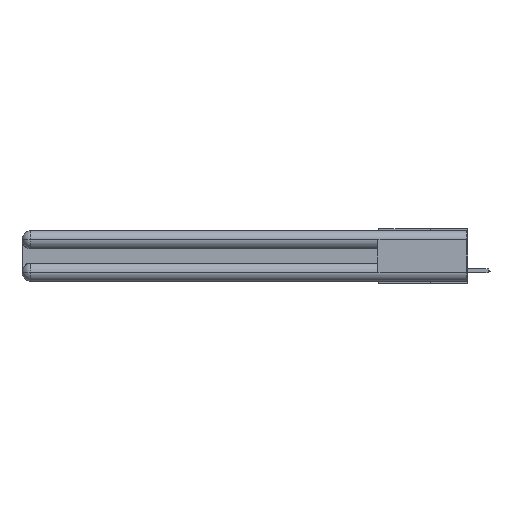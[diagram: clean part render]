
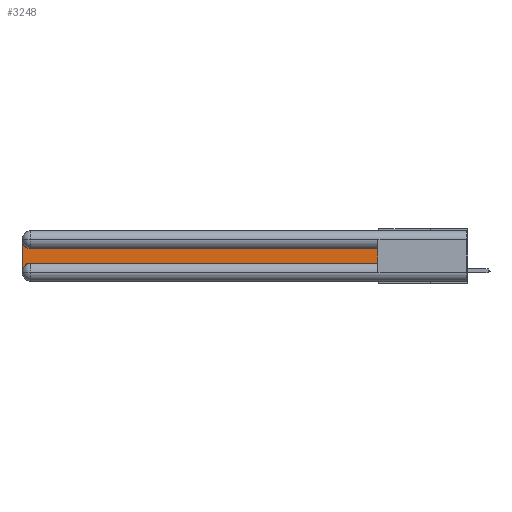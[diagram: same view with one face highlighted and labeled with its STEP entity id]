
A CAD part, left-side view. The second image highlights one B-rep face of the part: STEP entity #3248.
In plain terms, the highlighted planar face has unit normal (-1, 0, 0).
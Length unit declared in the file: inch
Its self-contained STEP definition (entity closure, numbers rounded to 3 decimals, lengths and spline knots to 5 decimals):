
#454 = CARTESIAN_POINT ( 'NONE',  ( 0.075, 3., -0.2775 ) ) ;
#665 = DIRECTION ( 'NONE',  ( 0., -1., 0. ) ) ;
#1036 = DIRECTION ( 'NONE',  ( 0., 1., 0. ) ) ;
#2066 = CARTESIAN_POINT ( 'NONE',  ( 0.075, 2.94, -0.1225 ) ) ;
#2293 = DIRECTION ( 'NONE',  ( 1., 0., 0. ) ) ;
#2367 = EDGE_CURVE ( 'NONE', #18410, #32623, #33781, .T. ) ;
#3248 = ADVANCED_FACE ( 'NONE', ( #12074 ), #4738, .F. ) ;
#3648 = CARTESIAN_POINT ( 'NONE',  ( 0.075, 2.94, -0.0625 ) ) ;
#4433 = DIRECTION ( 'NONE',  ( 0., 0., -1. ) ) ;
#4738 = PLANE ( 'NONE',  #27970 ) ;
#5517 = CARTESIAN_POINT ( 'NONE',  ( 0.075, 2.94, -0.2775 ) ) ;
#6351 = EDGE_CURVE ( 'NONE', #13117, #14638, #25207, .T. ) ;
#6501 = LINE ( 'NONE', #11069, #33966 ) ;
#7961 = CARTESIAN_POINT ( 'NONE',  ( 0.075, 0.6, -0.1225 ) ) ;
#9900 = CARTESIAN_POINT ( 'NONE',  ( 0.075, 3., -0.0625 ) ) ;
#10849 = LINE ( 'NONE', #24907, #33759 ) ;
#11069 = CARTESIAN_POINT ( 'NONE',  ( 0.075, 0.6, -0.2175 ) ) ;
#12074 = FACE_OUTER_BOUND ( 'NONE', #20539, .T. ) ;
#12689 = EDGE_CURVE ( 'NONE', #16022, #32002, #6501, .T. ) ;
#13117 = VERTEX_POINT ( 'NONE', #2066 ) ;
#13530 = ORIENTED_EDGE ( 'NONE', *, *, #12689, .T. ) ;
#14153 = VECTOR ( 'NONE', #27728, 39.37008 ) ;
#14638 = VERTEX_POINT ( 'NONE', #9900 ) ;
#15574 = CARTESIAN_POINT ( 'NONE',  ( 0.075, 3., -0.1225 ) ) ;
#16022 = VERTEX_POINT ( 'NONE', #25966 ) ;
#16686 = DIRECTION ( 'NONE',  ( 0., 0., 1. ) ) ;
#18410 = VERTEX_POINT ( 'NONE', #454 ) ;
#20134 = ORIENTED_EDGE ( 'NONE', *, *, #30797, .T. ) ;
#20539 = EDGE_LOOP ( 'NONE', ( #21805, #30813, #20134, #25543, #29751, #13530 ) ) ;
#21438 = DIRECTION ( 'NONE',  ( 0., 0., -1. ) ) ;
#21559 = DIRECTION ( 'NONE',  ( 1., 0., 0. ) ) ;
#21805 = ORIENTED_EDGE ( 'NONE', *, *, #28909, .T. ) ;
#23029 = VECTOR ( 'NONE', #665, 39.37008 ) ;
#23336 = DIRECTION ( 'NONE',  ( 0., 0., -1. ) ) ;
#24907 = CARTESIAN_POINT ( 'NONE',  ( 0.075, 0.6, -0.1225 ) ) ;
#25207 = CIRCLE ( 'NONE', #30865, 0.06 ) ;
#25400 = CARTESIAN_POINT ( 'NONE',  ( 0.075, 3., -0.2175 ) ) ;
#25543 = ORIENTED_EDGE ( 'NONE', *, *, #2367, .T. ) ;
#25966 = CARTESIAN_POINT ( 'NONE',  ( 0.075, 0.6, -0.2175 ) ) ;
#26603 = CARTESIAN_POINT ( 'NONE',  ( 0.075, 0.6, -0.2175 ) ) ;
#26721 = CARTESIAN_POINT ( 'NONE',  ( 0.075, 2.94, -0.2175 ) ) ;
#27628 = LINE ( 'NONE', #26603, #23029 ) ;
#27728 = DIRECTION ( 'NONE',  ( 0., 0., -1. ) ) ;
#27970 = AXIS2_PLACEMENT_3D ( 'NONE', #15574, #2293, #23336 ) ;
#28297 = DIRECTION ( 'NONE',  ( 1., 0., 0. ) ) ;
#28831 = AXIS2_PLACEMENT_3D ( 'NONE', #5517, #21559, #21438 ) ;
#28909 = EDGE_CURVE ( 'NONE', #32002, #13117, #10849, .T. ) ;
#29490 = LINE ( 'NONE', #25400, #14153 ) ;
#29751 = ORIENTED_EDGE ( 'NONE', *, *, #33095, .T. ) ;
#30797 = EDGE_CURVE ( 'NONE', #14638, #18410, #29490, .T. ) ;
#30813 = ORIENTED_EDGE ( 'NONE', *, *, #6351, .T. ) ;
#30865 = AXIS2_PLACEMENT_3D ( 'NONE', #3648, #28297, #4433 ) ;
#32002 = VERTEX_POINT ( 'NONE', #7961 ) ;
#32623 = VERTEX_POINT ( 'NONE', #26721 ) ;
#33095 = EDGE_CURVE ( 'NONE', #32623, #16022, #27628, .T. ) ;
#33759 = VECTOR ( 'NONE', #1036, 39.37008 ) ;
#33781 = CIRCLE ( 'NONE', #28831, 0.06 ) ;
#33966 = VECTOR ( 'NONE', #16686, 39.37008 ) ;
